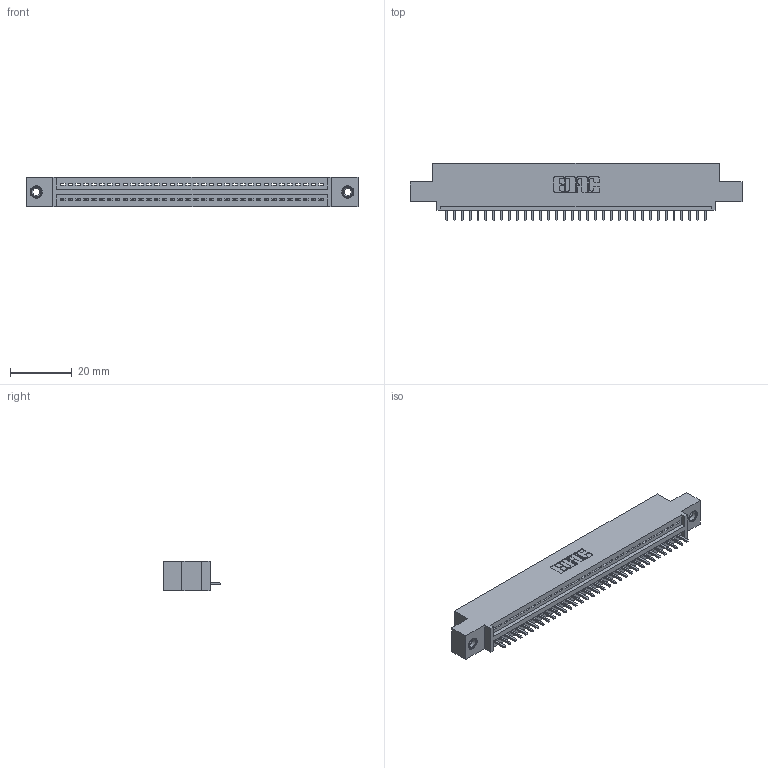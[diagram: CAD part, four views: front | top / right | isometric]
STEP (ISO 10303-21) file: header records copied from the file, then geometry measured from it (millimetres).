
FILE_DESCRIPTION (( 'STEP AP203' ), '1' );
FILE_NAME ('345-034-521-408.STEP', '2018-08-29T00:30:59', ( '' ), ( '' ), 'SwSTEP 2.0', 'SolidWorks 2016', '' );
FILE_SCHEMA (( 'CONFIG_CONTROL_DESIGN' ));
Length unit declared in the file: inch
Products named in the file (4): 345-292-001_345-293-121; 345-250-001_345-250-003-102; 345-034-521-408; 345 Part_0.110 Offset - 0.156 Dia-TI
Assembly tree (37 placements, depth 2):
  345-034-521-408
    345 Part_0.110 Offset - 0.156 Dia-TI
    345-292-001_345-293-121  x34
    345-250-001_345-250-003-102  x2
Bounding box: 107.57 x 18.72 x 9.4 mm (x, y, z)
Volume: 9974.9 mm3; surface area: 12869.7 mm2
Topology: 37 solids, 37 shells, 2162 faces, 6473 edges, 4262 vertices
Faces by surface type: plane 1476, cylinder 670, cone 12, torus 4
Entity records: 28002 total; most frequent: CARTESIAN_POINT 4833, ORIENTED_EDGE 4794, DIRECTION 4259, EDGE_CURVE 2397, VECTOR 2109, LINE 2109, VERTEX_POINT 1592, AXIS2_PLACEMENT_3D 1075
